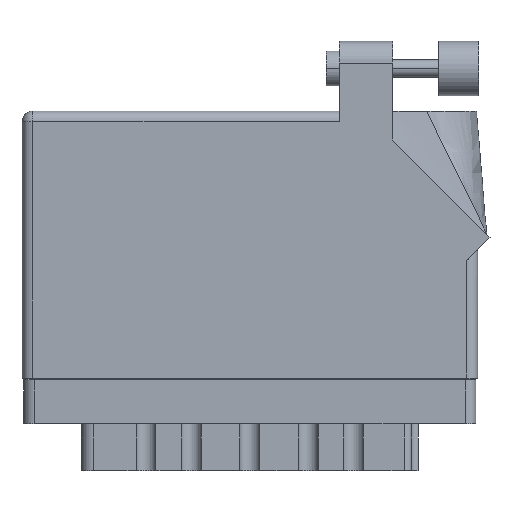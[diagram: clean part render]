
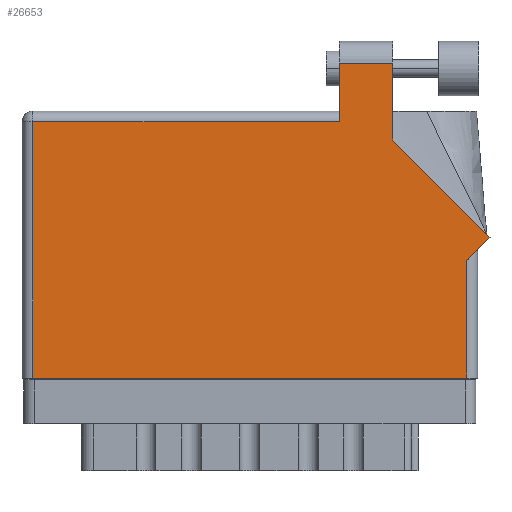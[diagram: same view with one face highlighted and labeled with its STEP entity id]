
A CAD part, front view. The second image highlights one B-rep face of the part: STEP entity #26653.
In plain terms, the highlighted face is planar.
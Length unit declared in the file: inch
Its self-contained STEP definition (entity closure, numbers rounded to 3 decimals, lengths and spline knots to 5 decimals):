
#220 = EDGE_CURVE ( 'NONE', #26511, #32764, #34901, .T. ) ;
#906 = PLANE ( 'NONE',  #13508 ) ;
#2175 = DIRECTION ( 'NONE',  ( 0.707, 0.707, 0. ) ) ;
#2196 = LINE ( 'NONE', #15088, #18982 ) ;
#2652 = DIRECTION ( 'NONE',  ( -0.707, 0.707, 0. ) ) ;
#3423 = LINE ( 'NONE', #14756, #8771 ) ;
#3799 = ORIENTED_EDGE ( 'NONE', *, *, #35524, .T. ) ;
#4670 = CARTESIAN_POINT ( 'NONE',  ( 2.55, 0., 0. ) ) ;
#6578 = VERTEX_POINT ( 'NONE', #41303 ) ;
#7094 = VERTEX_POINT ( 'NONE', #27753 ) ;
#8168 = ORIENTED_EDGE ( 'NONE', *, *, #220, .T. ) ;
#8771 = VECTOR ( 'NONE', #37929, 39.37008 ) ;
#9415 = CARTESIAN_POINT ( 'NONE',  ( 1.819, 1.805, 0. ) ) ;
#9522 = CARTESIAN_POINT ( 'NONE',  ( 2.55, 0.675, 0. ) ) ;
#9760 = EDGE_CURVE ( 'NONE', #47048, #6578, #34452, .T. ) ;
#9933 = ORIENTED_EDGE ( 'NONE', *, *, #21569, .T. ) ;
#10683 = DIRECTION ( 'NONE',  ( 1., 0., 0. ) ) ;
#11499 = VECTOR ( 'NONE', #2175, 39.37008 ) ;
#11735 = CARTESIAN_POINT ( 'NONE',  ( 2.68271, 0.80771, 0. ) ) ;
#12495 = VERTEX_POINT ( 'NONE', #45341 ) ;
#13508 = AXIS2_PLACEMENT_3D ( 'NONE', #31034, #35095, #39136 ) ;
#13865 = ORIENTED_EDGE ( 'NONE', *, *, #19054, .T. ) ;
#14362 = VECTOR ( 'NONE', #25836, 39.37008 ) ;
#14435 = LINE ( 'NONE', #48393, #23825 ) ;
#14756 = CARTESIAN_POINT ( 'NONE',  ( 0.062, 0., 0. ) ) ;
#15088 = CARTESIAN_POINT ( 'NONE',  ( 2.126, 1.36442, 0. ) ) ;
#18982 = VECTOR ( 'NONE', #44983, 39.37008 ) ;
#19054 = EDGE_CURVE ( 'NONE', #32764, #46280, #26331, .T. ) ;
#19772 = LINE ( 'NONE', #44310, #22732 ) ;
#21569 = EDGE_CURVE ( 'NONE', #25590, #7094, #2196, .T. ) ;
#21634 = EDGE_CURVE ( 'NONE', #12495, #26511, #3423, .T. ) ;
#22501 = CARTESIAN_POINT ( 'NONE',  ( 2.55, 0.737, 0. ) ) ;
#22732 = VECTOR ( 'NONE', #36731, 39.37008 ) ;
#22986 = VECTOR ( 'NONE', #38034, 39.37008 ) ;
#23825 = VECTOR ( 'NONE', #2652, 39.37008 ) ;
#25590 = VERTEX_POINT ( 'NONE', #46143 ) ;
#25836 = DIRECTION ( 'NONE',  ( 0., 1., 0. ) ) ;
#26331 = LINE ( 'NONE', #22501, #14362 ) ;
#26511 = VERTEX_POINT ( 'NONE', #38478 ) ;
#26653 = ADVANCED_FACE ( 'NONE', ( #33363 ), #906, .F. ) ;
#27428 = ORIENTED_EDGE ( 'NONE', *, *, #41433, .T. ) ;
#27753 = CARTESIAN_POINT ( 'NONE',  ( 2.126, 1.805, 0. ) ) ;
#29111 = EDGE_CURVE ( 'NONE', #46280, #40341, #35523, .T. ) ;
#29995 = VECTOR ( 'NONE', #34649, 39.37008 ) ;
#30439 = CARTESIAN_POINT ( 'NONE',  ( 1.819, 1.53, 0. ) ) ;
#30908 = EDGE_CURVE ( 'NONE', #40341, #25590, #14435, .T. ) ;
#31034 = CARTESIAN_POINT ( 'NONE',  ( 0., 1.53, 0. ) ) ;
#32764 = VERTEX_POINT ( 'NONE', #4670 ) ;
#33292 = ORIENTED_EDGE ( 'NONE', *, *, #29111, .T. ) ;
#33363 = FACE_OUTER_BOUND ( 'NONE', #44055, .T. ) ;
#33609 = LINE ( 'NONE', #34991, #29995 ) ;
#33784 = ORIENTED_EDGE ( 'NONE', *, *, #9760, .T. ) ;
#34452 = LINE ( 'NONE', #30439, #22986 ) ;
#34649 = DIRECTION ( 'NONE',  ( -1., 0., 0. ) ) ;
#34901 = LINE ( 'NONE', #37540, #46336 ) ;
#34991 = CARTESIAN_POINT ( 'NONE',  ( 1.819, 1.805, 0. ) ) ;
#35095 = DIRECTION ( 'NONE',  ( 0., 0., -1. ) ) ;
#35523 = LINE ( 'NONE', #40895, #11499 ) ;
#35524 = EDGE_CURVE ( 'NONE', #7094, #47048, #33609, .T. ) ;
#36731 = DIRECTION ( 'NONE',  ( -1., 0., 0. ) ) ;
#37540 = CARTESIAN_POINT ( 'NONE',  ( 0., 0., 0. ) ) ;
#37929 = DIRECTION ( 'NONE',  ( 0., -1., 0. ) ) ;
#38034 = DIRECTION ( 'NONE',  ( 0., -1., 0. ) ) ;
#38478 = CARTESIAN_POINT ( 'NONE',  ( 0.062, 0., 0. ) ) ;
#39136 = DIRECTION ( 'NONE',  ( -1., 0., 0. ) ) ;
#40341 = VERTEX_POINT ( 'NONE', #11735 ) ;
#40895 = CARTESIAN_POINT ( 'NONE',  ( 2.612, 0.737, 0. ) ) ;
#41303 = CARTESIAN_POINT ( 'NONE',  ( 1.819, 1.468, 0. ) ) ;
#41433 = EDGE_CURVE ( 'NONE', #6578, #12495, #19772, .T. ) ;
#44055 = EDGE_LOOP ( 'NONE', ( #9933, #3799, #33784, #27428, #47947, #8168, #13865, #33292, #47396 ) ) ;
#44310 = CARTESIAN_POINT ( 'NONE',  ( 0., 1.468, 0. ) ) ;
#44983 = DIRECTION ( 'NONE',  ( 0., 1., 0. ) ) ;
#45341 = CARTESIAN_POINT ( 'NONE',  ( 0.062, 1.468, 0. ) ) ;
#46143 = CARTESIAN_POINT ( 'NONE',  ( 2.126, 1.36442, 0. ) ) ;
#46280 = VERTEX_POINT ( 'NONE', #9522 ) ;
#46336 = VECTOR ( 'NONE', #10683, 39.37008 ) ;
#47048 = VERTEX_POINT ( 'NONE', #9415 ) ;
#47396 = ORIENTED_EDGE ( 'NONE', *, *, #30908, .T. ) ;
#47947 = ORIENTED_EDGE ( 'NONE', *, *, #21634, .T. ) ;
#48393 = CARTESIAN_POINT ( 'NONE',  ( 2.68271, 0.80771, 0. ) ) ;
